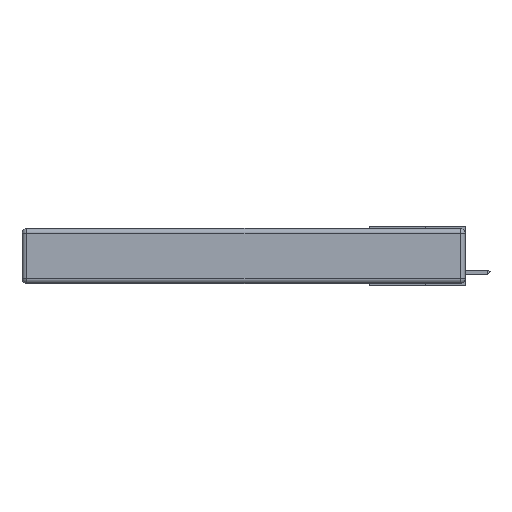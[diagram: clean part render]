
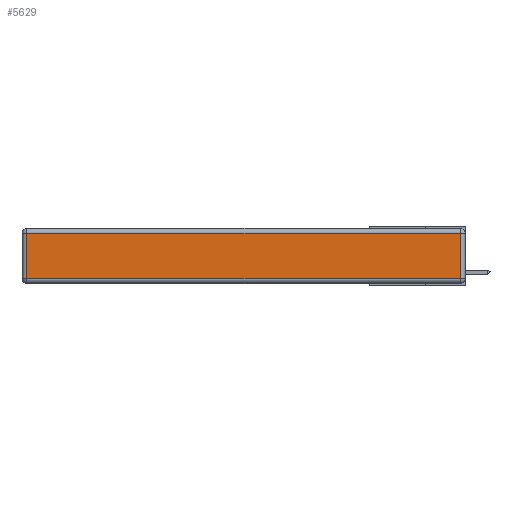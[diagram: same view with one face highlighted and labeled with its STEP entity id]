
A CAD part, left-side view. The second image highlights one B-rep face of the part: STEP entity #5629.
In plain terms, the highlighted planar face has unit normal (-1, 0, 0).
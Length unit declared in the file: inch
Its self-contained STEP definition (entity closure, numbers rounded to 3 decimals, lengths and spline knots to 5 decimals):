
#43 = VECTOR ( 'NONE', #4953, 39.37008 ) ;
#254 = VERTEX_POINT ( 'NONE', #3919 ) ;
#646 = CARTESIAN_POINT ( 'NONE',  ( 0., 0., -0.343 ) ) ;
#1770 = PLANE ( 'NONE',  #5721 ) ;
#2185 = CARTESIAN_POINT ( 'NONE',  ( 0., 2.75, -0.03 ) ) ;
#2483 = LINE ( 'NONE', #2185, #10613 ) ;
#2845 = DIRECTION ( 'NONE',  ( -1., 0., 0. ) ) ;
#3208 = CARTESIAN_POINT ( 'NONE',  ( 0., 0.03, -0.313 ) ) ;
#3290 = EDGE_CURVE ( 'NONE', #10328, #5861, #4342, .T. ) ;
#3919 = CARTESIAN_POINT ( 'NONE',  ( 0., 0.03, -0.03 ) ) ;
#4213 = ORIENTED_EDGE ( 'NONE', *, *, #5823, .T. ) ;
#4342 = LINE ( 'NONE', #7007, #43 ) ;
#4378 = CARTESIAN_POINT ( 'NONE',  ( 0., 2.72, -0.313 ) ) ;
#4953 = DIRECTION ( 'NONE',  ( 0., -1., 0. ) ) ;
#5070 = ORIENTED_EDGE ( 'NONE', *, *, #13388, .T. ) ;
#5096 = EDGE_LOOP ( 'NONE', ( #8432, #5070, #4213, #10636 ) ) ;
#5629 = ADVANCED_FACE ( 'NONE', ( #7288 ), #1770, .T. ) ;
#5721 = AXIS2_PLACEMENT_3D ( 'NONE', #646, #2845, #10266 ) ;
#5823 = EDGE_CURVE ( 'NONE', #254, #8048, #2483, .T. ) ;
#5861 = VERTEX_POINT ( 'NONE', #3208 ) ;
#6313 = DIRECTION ( 'NONE',  ( 0., 1., 0. ) ) ;
#6648 = VECTOR ( 'NONE', #13211, 39.37008 ) ;
#7007 = CARTESIAN_POINT ( 'NONE',  ( 0., 0., -0.313 ) ) ;
#7288 = FACE_OUTER_BOUND ( 'NONE', #5096, .T. ) ;
#8048 = VERTEX_POINT ( 'NONE', #9674 ) ;
#8388 = EDGE_CURVE ( 'NONE', #8048, #10328, #13343, .T. ) ;
#8432 = ORIENTED_EDGE ( 'NONE', *, *, #3290, .T. ) ;
#8632 = LINE ( 'NONE', #10166, #6648 ) ;
#9674 = CARTESIAN_POINT ( 'NONE',  ( 0., 2.72, -0.03 ) ) ;
#10166 = CARTESIAN_POINT ( 'NONE',  ( 0., 0.03, -0.343 ) ) ;
#10266 = DIRECTION ( 'NONE',  ( 0., 0., 1. ) ) ;
#10328 = VERTEX_POINT ( 'NONE', #4378 ) ;
#10613 = VECTOR ( 'NONE', #6313, 39.37008 ) ;
#10636 = ORIENTED_EDGE ( 'NONE', *, *, #8388, .T. ) ;
#11740 = DIRECTION ( 'NONE',  ( 0., 0., -1. ) ) ;
#12010 = VECTOR ( 'NONE', #11740, 39.37008 ) ;
#12667 = CARTESIAN_POINT ( 'NONE',  ( 0., 2.72, -0.343 ) ) ;
#13211 = DIRECTION ( 'NONE',  ( 0., 0., 1. ) ) ;
#13343 = LINE ( 'NONE', #12667, #12010 ) ;
#13388 = EDGE_CURVE ( 'NONE', #5861, #254, #8632, .T. ) ;
